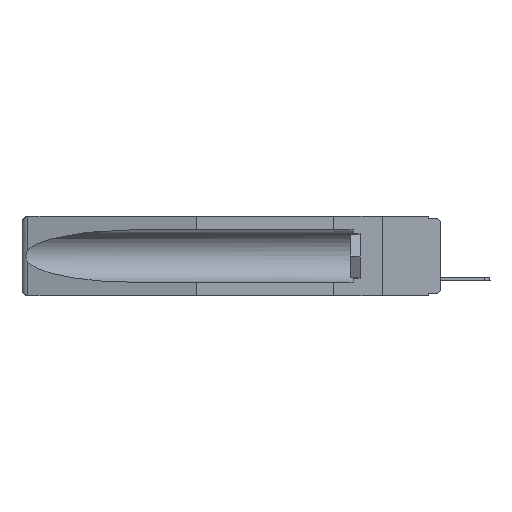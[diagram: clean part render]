
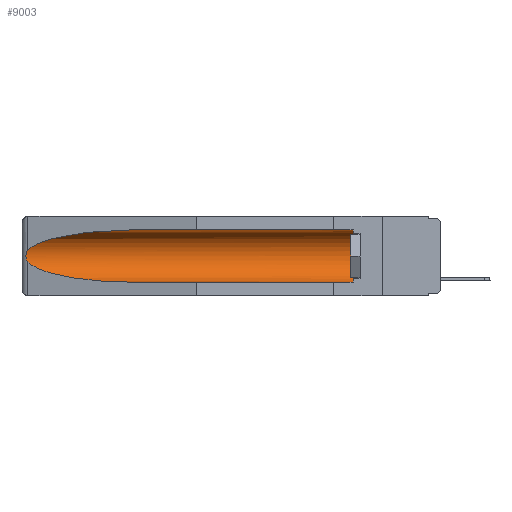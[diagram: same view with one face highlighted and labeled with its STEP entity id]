
A CAD part, left-side view. The second image highlights one B-rep face of the part: STEP entity #9003.
In plain terms, the highlighted cylindrical face has radius 2.857 mm (diameter 5.715 mm), a partial arc.
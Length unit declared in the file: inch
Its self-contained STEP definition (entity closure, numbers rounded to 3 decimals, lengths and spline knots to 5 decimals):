
#84 = DIRECTION ( 'NONE',  ( 0., -1., 0. ) ) ;
#217 = DIRECTION ( 'NONE',  ( 0., 1., 0. ) ) ;
#610 = CARTESIAN_POINT ( 'NONE',  ( 0.26537, 1.52718, -0.19328 ) ) ;
#854 = CARTESIAN_POINT ( 'NONE',  ( 0.2673, 1.53269, -0.17917 ) ) ;
#978 = CARTESIAN_POINT ( 'NONE',  ( 0.155, -0.30754, -0.284 ) ) ;
#984 = EDGE_CURVE ( 'NONE', #3239, #11703, #2623, .T. ) ;
#2346 = AXIS2_PLACEMENT_3D ( 'NONE', #8827, #84, #13420 ) ;
#2623 = LINE ( 'NONE', #10280, #10724 ) ;
#2915 = B_SPLINE_CURVE_WITH_KNOTS ( 'NONE', 3,
 ( #3270, #8360, #7203, #15985, #4439, #3436, #854, #6026, #8520, #610 ),
 .UNSPECIFIED., .F., .F.,
 ( 4, 2, 2, 2, 4 ),
 ( 0., 0.00029, 0.00058, 0.00087, 0.00117 ),
 .UNSPECIFIED. ) ;
#2921 = CARTESIAN_POINT ( 'NONE',  ( 0.155, 1.07973, -0.059 ) ) ;
#2968 = ORIENTED_EDGE ( 'NONE', *, *, #7924, .T. ) ;
#2979 = CARTESIAN_POINT ( 'NONE',  ( 0.155, 1.07973, -0.059 ) ) ;
#3239 = VERTEX_POINT ( 'NONE', #12554 ) ;
#3270 = CARTESIAN_POINT ( 'NONE',  ( 0.26537, 1.52718, -0.14972 ) ) ;
#3436 = CARTESIAN_POINT ( 'NONE',  ( 0.2675, 1.53308, -0.17534 ) ) ;
#3667 = VECTOR ( 'NONE', #5990, 39.37008 ) ;
#3690 = ORIENTED_EDGE ( 'NONE', *, *, #6556, .T. ) ;
#3920 = CARTESIAN_POINT ( 'NONE',  ( 0.155, 1.07973, -0.284 ) ) ;
#4043 = EDGE_LOOP ( 'NONE', ( #9675, #2968, #3690, #13654, #7908, #10710 ) ) ;
#4125 =( BOUNDED_CURVE ( )  B_SPLINE_CURVE ( 3, ( #5255, #10318, #15313, #3920 ),
 .UNSPECIFIED., .F., .F. ) 
 B_SPLINE_CURVE_WITH_KNOTS ( ( 4, 4 ),
 ( 0.1948, 1.5708 ),
 .UNSPECIFIED. ) 
 CURVE ( )  GEOMETRIC_REPRESENTATION_ITEM ( )  RATIONAL_B_SPLINE_CURVE ( ( 1., 0.848, 0.848, 1. ) ) 
 REPRESENTATION_ITEM ( '' )  );
#4439 = CARTESIAN_POINT ( 'NONE',  ( 0.2675, 1.53308, -0.16763 ) ) ;
#5255 = CARTESIAN_POINT ( 'NONE',  ( 0.26537, 1.52718, -0.19328 ) ) ;
#5905 = LINE ( 'NONE', #978, #3667 ) ;
#5990 = DIRECTION ( 'NONE',  ( 0., 1., 0. ) ) ;
#6026 = CARTESIAN_POINT ( 'NONE',  ( 0.26655, 1.53094, -0.18657 ) ) ;
#6504 = VERTEX_POINT ( 'NONE', #6761 ) ;
#6556 = EDGE_CURVE ( 'NONE', #12681, #6504, #4125, .T. ) ;
#6761 = CARTESIAN_POINT ( 'NONE',  ( 0.155, 1.07973, -0.284 ) ) ;
#7203 = CARTESIAN_POINT ( 'NONE',  ( 0.26654, 1.53092, -0.15636 ) ) ;
#7332 = CYLINDRICAL_SURFACE ( 'NONE', #13732, 0.1125 ) ;
#7451 = CARTESIAN_POINT ( 'NONE',  ( 0.26537, 1.52718, -0.14972 ) ) ;
#7677 = EDGE_CURVE ( 'NONE', #14847, #6504, #5905, .T. ) ;
#7908 = ORIENTED_EDGE ( 'NONE', *, *, #9803, .T. ) ;
#7924 = EDGE_CURVE ( 'NONE', #11119, #12681, #2915, .T. ) ;
#8360 = CARTESIAN_POINT ( 'NONE',  ( 0.26597, 1.52961, -0.15275 ) ) ;
#8520 = CARTESIAN_POINT ( 'NONE',  ( 0.26597, 1.5296, -0.19026 ) ) ;
#8561 = DIRECTION ( 'NONE',  ( 0., 1., 0. ) ) ;
#8827 = CARTESIAN_POINT ( 'NONE',  ( 0.155, 0.126, -0.1715 ) ) ;
#9003 = ADVANCED_FACE ( 'NONE', ( #11357 ), #7332, .F. ) ;
#9155 = CARTESIAN_POINT ( 'NONE',  ( 0.25451, 1.48313, -0.09465 ) ) ;
#9675 = ORIENTED_EDGE ( 'NONE', *, *, #13440, .T. ) ;
#9803 = EDGE_CURVE ( 'NONE', #14847, #3239, #12166, .T. ) ;
#10280 = CARTESIAN_POINT ( 'NONE',  ( 0.155, -0.30754, -0.059 ) ) ;
#10318 = CARTESIAN_POINT ( 'NONE',  ( 0.25451, 1.48313, -0.24835 ) ) ;
#10631 = CARTESIAN_POINT ( 'NONE',  ( 0.26537, 1.52718, -0.14972 ) ) ;
#10710 = ORIENTED_EDGE ( 'NONE', *, *, #984, .T. ) ;
#10724 = VECTOR ( 'NONE', #217, 39.37008 ) ;
#11119 = VERTEX_POINT ( 'NONE', #7451 ) ;
#11357 = FACE_OUTER_BOUND ( 'NONE', #4043, .T. ) ;
#11703 = VERTEX_POINT ( 'NONE', #2921 ) ;
#12166 = CIRCLE ( 'NONE', #2346, 0.1125 ) ;
#12309 = CARTESIAN_POINT ( 'NONE',  ( 0.26537, 1.52718, -0.19328 ) ) ;
#12554 = CARTESIAN_POINT ( 'NONE',  ( 0.155, 0.126, -0.059 ) ) ;
#12602 =( BOUNDED_CURVE ( )  B_SPLINE_CURVE ( 3, ( #2979, #15864, #9155, #10631 ),
 .UNSPECIFIED., .F., .F. ) 
 B_SPLINE_CURVE_WITH_KNOTS ( ( 4, 4 ),
 ( 4.71239, 6.08839 ),
 .UNSPECIFIED. ) 
 CURVE ( )  GEOMETRIC_REPRESENTATION_ITEM ( )  RATIONAL_B_SPLINE_CURVE ( ( 1., 0.848, 0.848, 1. ) ) 
 REPRESENTATION_ITEM ( '' )  );
#12681 = VERTEX_POINT ( 'NONE', #12309 ) ;
#13420 = DIRECTION ( 'NONE',  ( 0., 0., 1. ) ) ;
#13440 = EDGE_CURVE ( 'NONE', #11703, #11119, #12602, .T. ) ;
#13451 = CARTESIAN_POINT ( 'NONE',  ( 0.155, 0.126, -0.284 ) ) ;
#13654 = ORIENTED_EDGE ( 'NONE', *, *, #7677, .F. ) ;
#13698 = CARTESIAN_POINT ( 'NONE',  ( 0.155, -0.30754, -0.1715 ) ) ;
#13732 = AXIS2_PLACEMENT_3D ( 'NONE', #13698, #8561, #16436 ) ;
#14847 = VERTEX_POINT ( 'NONE', #13451 ) ;
#15313 = CARTESIAN_POINT ( 'NONE',  ( 0.21114, 1.30732, -0.284 ) ) ;
#15864 = CARTESIAN_POINT ( 'NONE',  ( 0.21114, 1.30732, -0.059 ) ) ;
#15985 = CARTESIAN_POINT ( 'NONE',  ( 0.2673, 1.5327, -0.16383 ) ) ;
#16436 = DIRECTION ( 'NONE',  ( 0., 0., 1. ) ) ;
